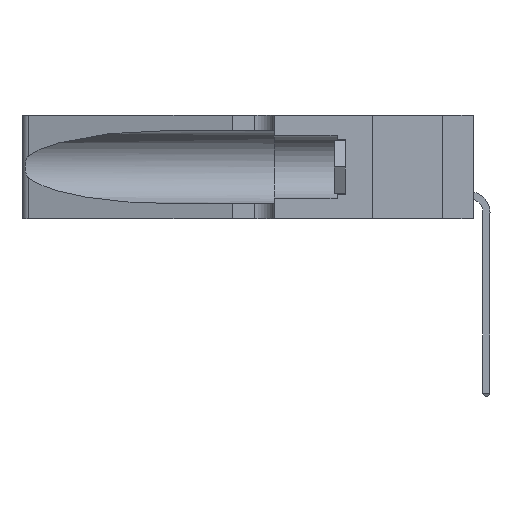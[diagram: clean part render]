
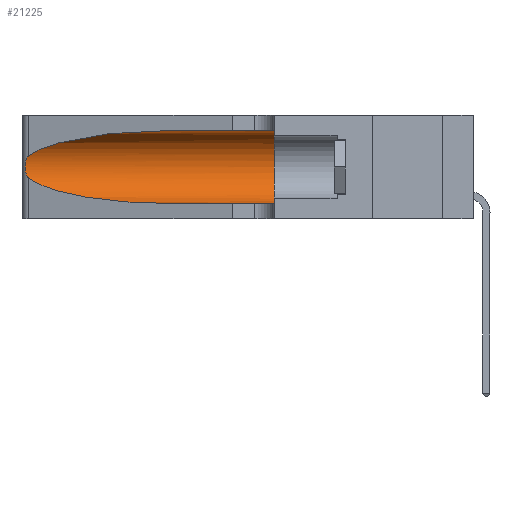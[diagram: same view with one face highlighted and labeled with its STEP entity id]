
A CAD part, left-side view. The second image highlights one B-rep face of the part: STEP entity #21225.
In plain terms, the highlighted cylindrical face has radius 3.308 mm (diameter 6.617 mm), a partial arc.
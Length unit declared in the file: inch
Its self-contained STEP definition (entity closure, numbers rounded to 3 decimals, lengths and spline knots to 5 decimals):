
#182 = CARTESIAN_POINT ( 'NONE',  ( 0.25487, 1.22718, 0.22369 ) ) ;
#464 = CARTESIAN_POINT ( 'NONE',  ( 0.1305, 0.72297, 0.31525 ) ) ;
#1000 = LINE ( 'NONE', #7907, #18908 ) ;
#1346 = CARTESIAN_POINT ( 'NONE',  ( 0.26075, 1.23896, 0.178 ) ) ;
#1461 = CARTESIAN_POINT ( 'NONE',  ( 0.25856, 1.23593, 0.16098 ) ) ;
#2202 =( BOUNDED_CURVE ( )  B_SPLINE_CURVE ( 3, ( #34196, #10363, #4752, #29040 ),
 .UNSPECIFIED., .F., .T. ) 
 B_SPLINE_CURVE_WITH_KNOTS ( ( 4, 4 ),
 ( 3.44316, 4.71239 ),
 .UNSPECIFIED. ) 
 CURVE ( )  GEOMETRIC_REPRESENTATION_ITEM ( )  RATIONAL_B_SPLINE_CURVE ( ( 1., 0.87, 0.87, 1. ) ) 
 REPRESENTATION_ITEM ( '' )  );
#2349 = DIRECTION ( 'NONE',  ( 0., -1., 0. ) ) ;
#3278 = EDGE_CURVE ( 'NONE', #17463, #26773, #18046, .T. ) ;
#4280 = ORIENTED_EDGE ( 'NONE', *, *, #16839, .F. ) ;
#4371 = CARTESIAN_POINT ( 'NONE',  ( 0.25487, 1.22718, 0.22369 ) ) ;
#4752 = CARTESIAN_POINT ( 'NONE',  ( 0.18966, 0.96281, 0.05475 ) ) ;
#6086 = DIRECTION ( 'NONE',  ( 0., 1., 0. ) ) ;
#6274 = CIRCLE ( 'NONE', #7692, 0.13025 ) ;
#6528 = EDGE_CURVE ( 'NONE', #17463, #10630, #1000, .T. ) ;
#7692 = AXIS2_PLACEMENT_3D ( 'NONE', #19271, #6086, #30278 ) ;
#7907 = CARTESIAN_POINT ( 'NONE',  ( 0.1305, 1.61858, 0.31525 ) ) ;
#8116 = CARTESIAN_POINT ( 'NONE',  ( 0.1305, 1.61858, 0.185 ) ) ;
#8715 = CARTESIAN_POINT ( 'NONE',  ( 0.1305, 0.35, 0.31525 ) ) ;
#9403 = CARTESIAN_POINT ( 'NONE',  ( 0.25639, 1.23186, 0.15144 ) ) ;
#10363 = CARTESIAN_POINT ( 'NONE',  ( 0.2373, 1.15595, 0.08982 ) ) ;
#10630 = VERTEX_POINT ( 'NONE', #8715 ) ;
#10785 = CARTESIAN_POINT ( 'NONE',  ( 0.25487, 1.22718, 0.14631 ) ) ;
#11142 = DIRECTION ( 'NONE',  ( 0., 0., -1. ) ) ;
#12426 = VECTOR ( 'NONE', #2349, 39.37008 ) ;
#12520 = EDGE_CURVE ( 'NONE', #27871, #18440, #24067, .T. ) ;
#13002 = CARTESIAN_POINT ( 'NONE',  ( 0.1305, 0.72297, 0.31525 ) ) ;
#13282 = VERTEX_POINT ( 'NONE', #10785 ) ;
#13443 = DIRECTION ( 'NONE',  ( 0., -1., 0. ) ) ;
#13850 = CARTESIAN_POINT ( 'NONE',  ( 0.2373, 1.15595, 0.28018 ) ) ;
#14834 = CARTESIAN_POINT ( 'NONE',  ( 0.26017, 1.23833, 0.17102 ) ) ;
#15780 = CARTESIAN_POINT ( 'NONE',  ( 0.1305, 0.72297, 0.05475 ) ) ;
#16839 = EDGE_CURVE ( 'NONE', #10630, #18440, #6274, .T. ) ;
#17435 = ORIENTED_EDGE ( 'NONE', *, *, #3278, .T. ) ;
#17438 = CARTESIAN_POINT ( 'NONE',  ( 0.26075, 1.23896, 0.19203 ) ) ;
#17463 = VERTEX_POINT ( 'NONE', #13002 ) ;
#18046 =( BOUNDED_CURVE ( )  B_SPLINE_CURVE ( 3, ( #464, #21832, #13850, #32571 ),
 .UNSPECIFIED., .F., .F. ) 
 B_SPLINE_CURVE_WITH_KNOTS ( ( 4, 4 ),
 ( 1.5708, 2.84003 ),
 .UNSPECIFIED. ) 
 CURVE ( )  GEOMETRIC_REPRESENTATION_ITEM ( )  RATIONAL_B_SPLINE_CURVE ( ( 1., 0.87, 0.87, 1. ) ) 
 REPRESENTATION_ITEM ( '' )  );
#18440 = VERTEX_POINT ( 'NONE', #24553 ) ;
#18868 = ORIENTED_EDGE ( 'NONE', *, *, #6528, .F. ) ;
#18908 = VECTOR ( 'NONE', #25277, 39.37008 ) ;
#19271 = CARTESIAN_POINT ( 'NONE',  ( 0.1305, 0.35, 0.185 ) ) ;
#19341 = AXIS2_PLACEMENT_3D ( 'NONE', #8116, #13443, #11142 ) ;
#19707 = ORIENTED_EDGE ( 'NONE', *, *, #12520, .T. ) ;
#19921 = EDGE_LOOP ( 'NONE', ( #17435, #26870, #31609, #19707, #4280, #18868 ) ) ;
#19968 = CARTESIAN_POINT ( 'NONE',  ( 0.25789, 1.23486, 0.15765 ) ) ;
#20326 = CARTESIAN_POINT ( 'NONE',  ( 0.25555, 1.22994, 0.2215 ) ) ;
#21027 = EDGE_CURVE ( 'NONE', #26773, #13282, #31736, .T. ) ;
#21225 = ADVANCED_FACE ( 'NONE', ( #24771 ), #24317, .F. ) ;
#21832 = CARTESIAN_POINT ( 'NONE',  ( 0.18966, 0.96281, 0.31525 ) ) ;
#22819 = CARTESIAN_POINT ( 'NONE',  ( 0.25854, 1.2359, 0.20912 ) ) ;
#24067 = LINE ( 'NONE', #26707, #12426 ) ;
#24317 = CYLINDRICAL_SURFACE ( 'NONE', #19341, 0.13025 ) ;
#24553 = CARTESIAN_POINT ( 'NONE',  ( 0.1305, 0.35, 0.05475 ) ) ;
#24771 = FACE_OUTER_BOUND ( 'NONE', #19921, .T. ) ;
#25277 = DIRECTION ( 'NONE',  ( 0., -1., 0. ) ) ;
#25723 = CARTESIAN_POINT ( 'NONE',  ( 0.25487, 1.22718, 0.14631 ) ) ;
#26707 = CARTESIAN_POINT ( 'NONE',  ( 0.1305, 1.61858, 0.05475 ) ) ;
#26773 = VERTEX_POINT ( 'NONE', #182 ) ;
#26870 = ORIENTED_EDGE ( 'NONE', *, *, #21027, .T. ) ;
#27871 = VERTEX_POINT ( 'NONE', #15780 ) ;
#28061 = CARTESIAN_POINT ( 'NONE',  ( 0.25555, 1.22993, 0.14849 ) ) ;
#28297 = CARTESIAN_POINT ( 'NONE',  ( 0.25787, 1.23484, 0.2124 ) ) ;
#29040 = CARTESIAN_POINT ( 'NONE',  ( 0.1305, 0.72297, 0.05475 ) ) ;
#30278 = DIRECTION ( 'NONE',  ( 0., 0., 1. ) ) ;
#30399 = EDGE_CURVE ( 'NONE', #13282, #27871, #2202, .T. ) ;
#31239 = CARTESIAN_POINT ( 'NONE',  ( 0.25639, 1.23184, 0.21858 ) ) ;
#31609 = ORIENTED_EDGE ( 'NONE', *, *, #30399, .T. ) ;
#31736 = B_SPLINE_CURVE_WITH_KNOTS ( 'NONE', 3,
 ( #4371, #20326, #31239, #28297, #22819, #33449, #17438, #1346, #14834, #1461, #19968, #9403, #28061, #25723 ),
 .UNSPECIFIED., .F., .F.,
 ( 4, 2, 2, 2, 2, 2, 4 ),
 ( 0., 0.00027, 0.00053, 0.00107, 0.0016, 0.00187, 0.00214 ),
 .UNSPECIFIED. ) ;
#32571 = CARTESIAN_POINT ( 'NONE',  ( 0.25487, 1.22718, 0.22369 ) ) ;
#33449 = CARTESIAN_POINT ( 'NONE',  ( 0.26018, 1.23835, 0.19895 ) ) ;
#34196 = CARTESIAN_POINT ( 'NONE',  ( 0.25487, 1.22718, 0.14631 ) ) ;
